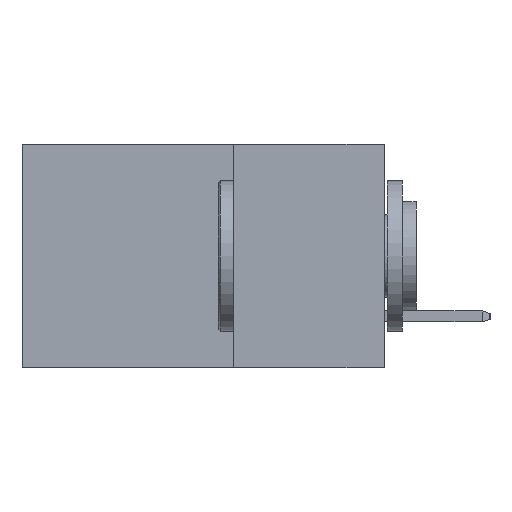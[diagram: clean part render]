
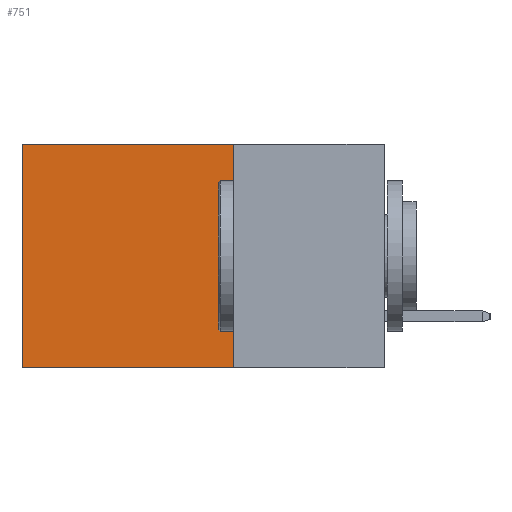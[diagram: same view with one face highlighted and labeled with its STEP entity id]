
A CAD part, left-side view. The second image highlights one B-rep face of the part: STEP entity #751.
In plain terms, the highlighted planar face has unit normal (-1, 0, 0).
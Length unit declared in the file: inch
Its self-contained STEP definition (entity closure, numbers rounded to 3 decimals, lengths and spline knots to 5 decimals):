
#119 = DIRECTION ( 'NONE',  ( 0., 1., 0. ) ) ;
#156 = VECTOR ( 'NONE', #4646, 39.37008 ) ;
#453 = CARTESIAN_POINT ( 'NONE',  ( 0.2615, 0.25, -0.37 ) ) ;
#730 = FACE_OUTER_BOUND ( 'NONE', #12226, .T. ) ;
#751 = ADVANCED_FACE ( 'NONE', ( #730 ), #13843, .F. ) ;
#1185 = DIRECTION ( 'NONE',  ( 0., 1., 0. ) ) ;
#1464 = CARTESIAN_POINT ( 'NONE',  ( 0.2615, 0.6, -0.37 ) ) ;
#1544 = VERTEX_POINT ( 'NONE', #16580 ) ;
#3979 = LINE ( 'NONE', #6571, #15524 ) ;
#4646 = DIRECTION ( 'NONE',  ( 0., 0., -1. ) ) ;
#5938 = ORIENTED_EDGE ( 'NONE', *, *, #16825, .F. ) ;
#6254 = AXIS2_PLACEMENT_3D ( 'NONE', #453, #7782, #11383 ) ;
#6571 = CARTESIAN_POINT ( 'NONE',  ( 0.2615, 0.25, 0. ) ) ;
#7782 = DIRECTION ( 'NONE',  ( 1., 0., 0. ) ) ;
#8245 = LINE ( 'NONE', #1464, #156 ) ;
#8289 = VECTOR ( 'NONE', #1185, 39.37008 ) ;
#8425 = ORIENTED_EDGE ( 'NONE', *, *, #16390, .T. ) ;
#9201 = CARTESIAN_POINT ( 'NONE',  ( 0.2615, 0.25, -0.37 ) ) ;
#9594 = VERTEX_POINT ( 'NONE', #14988 ) ;
#10509 = EDGE_CURVE ( 'NONE', #18061, #1544, #12889, .T. ) ;
#10757 = CARTESIAN_POINT ( 'NONE',  ( 0.2615, 0.25, -0.37 ) ) ;
#10914 = VECTOR ( 'NONE', #12302, 39.37008 ) ;
#11234 = ORIENTED_EDGE ( 'NONE', *, *, #11335, .T. ) ;
#11335 = EDGE_CURVE ( 'NONE', #16849, #1544, #8245, .T. ) ;
#11383 = DIRECTION ( 'NONE',  ( 0., 0., -1. ) ) ;
#12226 = EDGE_LOOP ( 'NONE', ( #11234, #13688, #5938, #8425 ) ) ;
#12302 = DIRECTION ( 'NONE',  ( 0., 0., -1. ) ) ;
#12363 = CARTESIAN_POINT ( 'NONE',  ( 0.2615, 0.6, 0. ) ) ;
#12889 = LINE ( 'NONE', #10757, #8289 ) ;
#13688 = ORIENTED_EDGE ( 'NONE', *, *, #10509, .F. ) ;
#13843 = PLANE ( 'NONE',  #6254 ) ;
#14988 = CARTESIAN_POINT ( 'NONE',  ( 0.2615, 0.25, 0. ) ) ;
#15033 = LINE ( 'NONE', #9201, #10914 ) ;
#15524 = VECTOR ( 'NONE', #119, 39.37008 ) ;
#16390 = EDGE_CURVE ( 'NONE', #9594, #16849, #3979, .T. ) ;
#16580 = CARTESIAN_POINT ( 'NONE',  ( 0.2615, 0.6, -0.37 ) ) ;
#16825 = EDGE_CURVE ( 'NONE', #9594, #18061, #15033, .T. ) ;
#16849 = VERTEX_POINT ( 'NONE', #12363 ) ;
#18061 = VERTEX_POINT ( 'NONE', #18302 ) ;
#18302 = CARTESIAN_POINT ( 'NONE',  ( 0.2615, 0.25, -0.37 ) ) ;
